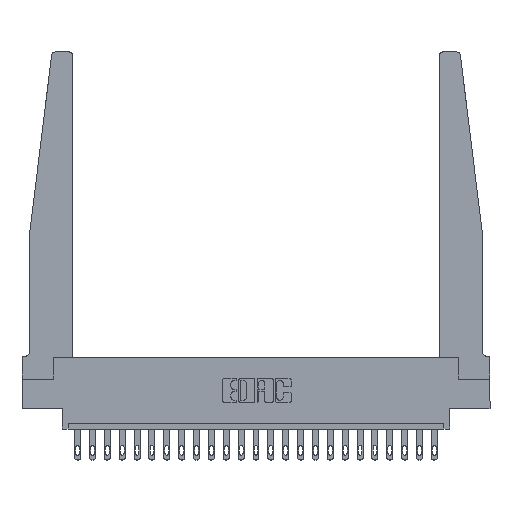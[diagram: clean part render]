
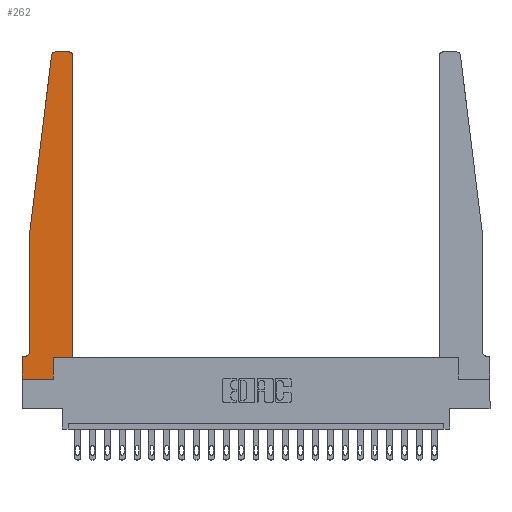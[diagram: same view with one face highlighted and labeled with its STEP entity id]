
A CAD part, top view. The second image highlights one B-rep face of the part: STEP entity #262.
In plain terms, the highlighted planar face has unit normal (0, 0, 1).
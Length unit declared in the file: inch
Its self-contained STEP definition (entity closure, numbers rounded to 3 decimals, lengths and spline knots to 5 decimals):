
#80 = LINE ( 'NONE', #12763, #21770 ) ;
#122 = CARTESIAN_POINT ( 'NONE',  ( 0., 0.1875, 0.37 ) ) ;
#172 = ORIENTED_EDGE ( 'NONE', *, *, #6131, .T. ) ;
#262 = ADVANCED_FACE ( 'NONE', ( #16291 ), #3835, .T. ) ;
#723 = VERTEX_POINT ( 'NONE', #8934 ) ;
#825 = EDGE_LOOP ( 'NONE', ( #15596, #10669, #11617, #8473, #9864, #172, #7576, #22091, #1977, #19937, #15146, #4825 ) ) ;
#1157 = CARTESIAN_POINT ( 'NONE',  ( 0.425, 0.18, 0.37 ) ) ;
#1336 = EDGE_CURVE ( 'NONE', #723, #14415, #17847, .T. ) ;
#1865 = LINE ( 'NONE', #21676, #16022 ) ;
#1872 = CARTESIAN_POINT ( 'NONE',  ( 0.25, 2.75, 0.37 ) ) ;
#1968 = LINE ( 'NONE', #3837, #8856 ) ;
#1977 = ORIENTED_EDGE ( 'NONE', *, *, #19009, .T. ) ;
#2079 = DIRECTION ( 'NONE',  ( 0., 0., 1. ) ) ;
#2310 = CARTESIAN_POINT ( 'NONE',  ( 0., 0., 0.37 ) ) ;
#2343 = LINE ( 'NONE', #9102, #22789 ) ;
#2919 = LINE ( 'NONE', #13757, #15647 ) ;
#3398 = DIRECTION ( 'NONE',  ( 0., 1., 0. ) ) ;
#3835 = PLANE ( 'NONE',  #17783 ) ;
#3837 = CARTESIAN_POINT ( 'NONE',  ( 0.065, 1.25, 0.37 ) ) ;
#4091 = VECTOR ( 'NONE', #12731, 39.37008 ) ;
#4147 = AXIS2_PLACEMENT_3D ( 'NONE', #20284, #13043, #9666 ) ;
#4279 = AXIS2_PLACEMENT_3D ( 'NONE', #14295, #9276, #16271 ) ;
#4323 = VERTEX_POINT ( 'NONE', #9905 ) ;
#4426 = CIRCLE ( 'NONE', #14105, 0.03 ) ;
#4689 = VERTEX_POINT ( 'NONE', #12205 ) ;
#4825 = ORIENTED_EDGE ( 'NONE', *, *, #10178, .T. ) ;
#4975 = VERTEX_POINT ( 'NONE', #11221 ) ;
#5246 = VECTOR ( 'NONE', #22284, 39.37008 ) ;
#5457 = CARTESIAN_POINT ( 'NONE',  ( 0.24675, 2.72367, 0.37 ) ) ;
#5672 = VERTEX_POINT ( 'NONE', #8367 ) ;
#6131 = EDGE_CURVE ( 'NONE', #5672, #20228, #2343, .T. ) ;
#6299 = CARTESIAN_POINT ( 'NONE',  ( 0.065, 0.2375, 0.37 ) ) ;
#6497 = EDGE_CURVE ( 'NONE', #21626, #9757, #1968, .T. ) ;
#6966 = EDGE_CURVE ( 'NONE', #14415, #11590, #4426, .T. ) ;
#7282 = DIRECTION ( 'NONE',  ( 0., 0., 1. ) ) ;
#7404 = DIRECTION ( 'NONE',  ( 1., 0., 0. ) ) ;
#7523 = CARTESIAN_POINT ( 'NONE',  ( 0.27653, 2.72, 0.37 ) ) ;
#7576 = ORIENTED_EDGE ( 'NONE', *, *, #8070, .T. ) ;
#8070 = EDGE_CURVE ( 'NONE', #20228, #11772, #80, .T. ) ;
#8080 = CARTESIAN_POINT ( 'NONE',  ( 0.425, 2.72, 0.37 ) ) ;
#8148 = EDGE_CURVE ( 'NONE', #9757, #5672, #14310, .T. ) ;
#8367 = CARTESIAN_POINT ( 'NONE',  ( 0.015, 0.1875, 0.37 ) ) ;
#8473 = ORIENTED_EDGE ( 'NONE', *, *, #6497, .T. ) ;
#8756 = VERTEX_POINT ( 'NONE', #8080 ) ;
#8856 = VECTOR ( 'NONE', #9185, 39.37008 ) ;
#8934 = CARTESIAN_POINT ( 'NONE',  ( 0.395, 2.75, 0.37 ) ) ;
#9102 = CARTESIAN_POINT ( 'NONE',  ( 0.065, 0.1875, 0.37 ) ) ;
#9183 = DIRECTION ( 'NONE',  ( 1., 0., 0. ) ) ;
#9185 = DIRECTION ( 'NONE',  ( 0., -1., 0. ) ) ;
#9276 = DIRECTION ( 'NONE',  ( 0., 0., -1. ) ) ;
#9325 = DIRECTION ( 'NONE',  ( -1., 0., 0. ) ) ;
#9666 = DIRECTION ( 'NONE',  ( 1., 0., 0. ) ) ;
#9757 = VERTEX_POINT ( 'NONE', #6299 ) ;
#9864 = ORIENTED_EDGE ( 'NONE', *, *, #8148, .T. ) ;
#9905 = CARTESIAN_POINT ( 'NONE',  ( 0.2605, 0., 0.37 ) ) ;
#10021 = DIRECTION ( 'NONE',  ( 1., 0., 0. ) ) ;
#10178 = EDGE_CURVE ( 'NONE', #8756, #723, #17169, .T. ) ;
#10316 = EDGE_CURVE ( 'NONE', #11772, #4323, #2919, .T. ) ;
#10669 = ORIENTED_EDGE ( 'NONE', *, *, #6966, .T. ) ;
#11138 = DIRECTION ( 'NONE',  ( 0., -1., 0. ) ) ;
#11221 = CARTESIAN_POINT ( 'NONE',  ( 0.2605, 0.18, 0.37 ) ) ;
#11590 = VERTEX_POINT ( 'NONE', #5457 ) ;
#11617 = ORIENTED_EDGE ( 'NONE', *, *, #18644, .T. ) ;
#11772 = VERTEX_POINT ( 'NONE', #2310 ) ;
#12114 = LINE ( 'NONE', #1157, #19795 ) ;
#12205 = CARTESIAN_POINT ( 'NONE',  ( 0.425, 0.18, 0.37 ) ) ;
#12470 = DIRECTION ( 'NONE',  ( -1., 0., 0. ) ) ;
#12731 = DIRECTION ( 'NONE',  ( 1., 0., 0. ) ) ;
#12763 = CARTESIAN_POINT ( 'NONE',  ( 0., 0., 0.37 ) ) ;
#13043 = DIRECTION ( 'NONE',  ( 0., 0., 1. ) ) ;
#13623 = DIRECTION ( 'NONE',  ( 0., 1., 0. ) ) ;
#13757 = CARTESIAN_POINT ( 'NONE',  ( 0., 0., 0.37 ) ) ;
#14105 = AXIS2_PLACEMENT_3D ( 'NONE', #7523, #7282, #7404 ) ;
#14295 = CARTESIAN_POINT ( 'NONE',  ( 0.015, 0.2375, 0.37 ) ) ;
#14310 = CIRCLE ( 'NONE', #4279, 0.05 ) ;
#14415 = VERTEX_POINT ( 'NONE', #19839 ) ;
#14702 = LINE ( 'NONE', #14816, #5246 ) ;
#14816 = CARTESIAN_POINT ( 'NONE',  ( 0.065, 1.25, 0.37 ) ) ;
#15146 = ORIENTED_EDGE ( 'NONE', *, *, #20474, .T. ) ;
#15596 = ORIENTED_EDGE ( 'NONE', *, *, #1336, .T. ) ;
#15647 = VECTOR ( 'NONE', #10021, 39.37008 ) ;
#16022 = VECTOR ( 'NONE', #3398, 39.37008 ) ;
#16271 = DIRECTION ( 'NONE',  ( -1., 0., 0. ) ) ;
#16291 = FACE_OUTER_BOUND ( 'NONE', #825, .T. ) ;
#16324 = CARTESIAN_POINT ( 'NONE',  ( 0.065, 1.25, 0.37 ) ) ;
#17169 = CIRCLE ( 'NONE', #4147, 0.03 ) ;
#17783 = AXIS2_PLACEMENT_3D ( 'NONE', #18065, #2079, #9183 ) ;
#17847 = LINE ( 'NONE', #1872, #22286 ) ;
#18064 = EDGE_CURVE ( 'NONE', #4975, #4689, #21508, .T. ) ;
#18065 = CARTESIAN_POINT ( 'NONE',  ( 0., 0.1875, 0.37 ) ) ;
#18644 = EDGE_CURVE ( 'NONE', #11590, #21626, #14702, .T. ) ;
#19009 = EDGE_CURVE ( 'NONE', #4323, #4975, #1865, .T. ) ;
#19530 = CARTESIAN_POINT ( 'NONE',  ( 0.425, 0.18, 0.37 ) ) ;
#19795 = VECTOR ( 'NONE', #13623, 39.37008 ) ;
#19839 = CARTESIAN_POINT ( 'NONE',  ( 0.27653, 2.75, 0.37 ) ) ;
#19937 = ORIENTED_EDGE ( 'NONE', *, *, #18064, .T. ) ;
#20228 = VERTEX_POINT ( 'NONE', #122 ) ;
#20284 = CARTESIAN_POINT ( 'NONE',  ( 0.395, 2.72, 0.37 ) ) ;
#20474 = EDGE_CURVE ( 'NONE', #4689, #8756, #12114, .T. ) ;
#21508 = LINE ( 'NONE', #19530, #4091 ) ;
#21626 = VERTEX_POINT ( 'NONE', #16324 ) ;
#21676 = CARTESIAN_POINT ( 'NONE',  ( 0.2605, 0.18, 0.37 ) ) ;
#21770 = VECTOR ( 'NONE', #11138, 39.37008 ) ;
#22091 = ORIENTED_EDGE ( 'NONE', *, *, #10316, .T. ) ;
#22284 = DIRECTION ( 'NONE',  ( -0.122, -0.992, 0. ) ) ;
#22286 = VECTOR ( 'NONE', #12470, 39.37008 ) ;
#22789 = VECTOR ( 'NONE', #9325, 39.37008 ) ;
